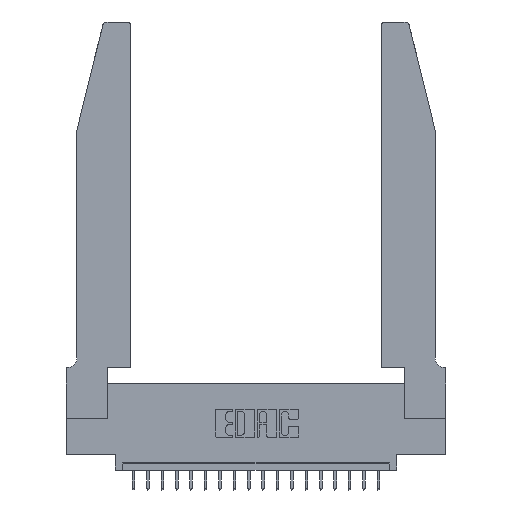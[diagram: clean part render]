
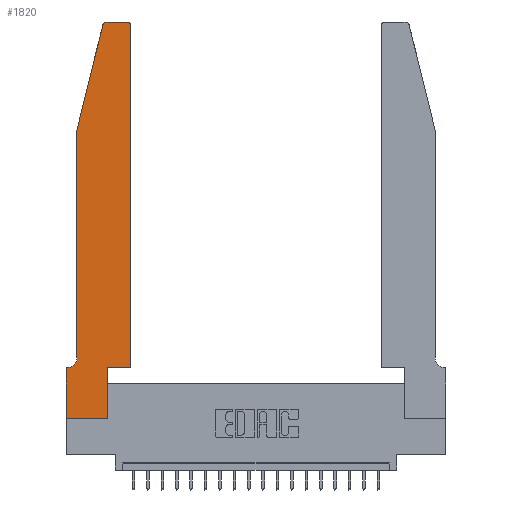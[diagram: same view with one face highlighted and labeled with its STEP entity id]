
A CAD part, top view. The second image highlights one B-rep face of the part: STEP entity #1820.
In plain terms, the highlighted planar face has unit normal (0, 0, 1).
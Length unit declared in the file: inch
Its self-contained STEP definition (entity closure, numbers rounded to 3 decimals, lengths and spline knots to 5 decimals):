
#83 = CARTESIAN_POINT ( 'NONE',  ( 0., 0., 0.37 ) ) ;
#143 = CARTESIAN_POINT ( 'NONE',  ( 0., 0.35, 0.37 ) ) ;
#421 = CARTESIAN_POINT ( 'NONE',  ( 0.0755, 0.42, 0.37 ) ) ;
#823 = CARTESIAN_POINT ( 'NONE',  ( 0.2605, 2.75, 0.37 ) ) ;
#1462 = VECTOR ( 'NONE', #4041, 39.37008 ) ;
#1718 = ORIENTED_EDGE ( 'NONE', *, *, #9220, .T. ) ;
#1743 = LINE ( 'NONE', #6698, #9475 ) ;
#1820 = ADVANCED_FACE ( 'NONE', ( #16213 ), #4867, .T. ) ;
#1913 = ORIENTED_EDGE ( 'NONE', *, *, #7084, .T. ) ;
#1983 = CARTESIAN_POINT ( 'NONE',  ( 0.2865, 0.35, 0.37 ) ) ;
#2235 = CARTESIAN_POINT ( 'NONE',  ( 0.284, 2.72, 0.37 ) ) ;
#2247 = VERTEX_POINT ( 'NONE', #15084 ) ;
#2311 = CARTESIAN_POINT ( 'NONE',  ( 0., 0., 0.37 ) ) ;
#2673 = AXIS2_PLACEMENT_3D ( 'NONE', #14909, #11725, #10182 ) ;
#2847 = CARTESIAN_POINT ( 'NONE',  ( 0.4505, 0.35, 0.37 ) ) ;
#3314 = ORIENTED_EDGE ( 'NONE', *, *, #6901, .T. ) ;
#3519 = VERTEX_POINT ( 'NONE', #1983 ) ;
#3571 = VECTOR ( 'NONE', #21142, 39.37008 ) ;
#3881 = CARTESIAN_POINT ( 'NONE',  ( 0.4505, 0.35, 0.37 ) ) ;
#4041 = DIRECTION ( 'NONE',  ( -1., 0., 0. ) ) ;
#4102 = CARTESIAN_POINT ( 'NONE',  ( 0.2865, 0., 0.37 ) ) ;
#4255 = CARTESIAN_POINT ( 'NONE',  ( 0.0055, 0.35, 0.37 ) ) ;
#4302 = LINE ( 'NONE', #5862, #3571 ) ;
#4397 = VERTEX_POINT ( 'NONE', #13463 ) ;
#4502 = CARTESIAN_POINT ( 'NONE',  ( 0.25487, 2.72718, 0.37 ) ) ;
#4761 = CARTESIAN_POINT ( 'NONE',  ( 0.0055, 0.42, 0.37 ) ) ;
#4792 = EDGE_CURVE ( 'NONE', #20558, #2247, #1743, .T. ) ;
#4867 = PLANE ( 'NONE',  #11579 ) ;
#5631 = VERTEX_POINT ( 'NONE', #143 ) ;
#5745 = LINE ( 'NONE', #7727, #11145 ) ;
#5862 = CARTESIAN_POINT ( 'NONE',  ( 0., 0., 0.37 ) ) ;
#5987 = DIRECTION ( 'NONE',  ( -1., 0., 0. ) ) ;
#6522 = VERTEX_POINT ( 'NONE', #421 ) ;
#6698 = CARTESIAN_POINT ( 'NONE',  ( 0.0755, 2., 0.37 ) ) ;
#6895 = EDGE_CURVE ( 'NONE', #7640, #20558, #8828, .T. ) ;
#6901 = EDGE_CURVE ( 'NONE', #14766, #4397, #20722, .T. ) ;
#7055 = ORIENTED_EDGE ( 'NONE', *, *, #10896, .T. ) ;
#7084 = EDGE_CURVE ( 'NONE', #19319, #17092, #4302, .T. ) ;
#7640 = VERTEX_POINT ( 'NONE', #21561 ) ;
#7681 = LINE ( 'NONE', #14392, #1462 ) ;
#7727 = CARTESIAN_POINT ( 'NONE',  ( 0.0755, 2., 0.37 ) ) ;
#7850 = DIRECTION ( 'NONE',  ( 0., 0., 1. ) ) ;
#7981 = ORIENTED_EDGE ( 'NONE', *, *, #12737, .T. ) ;
#8828 = CIRCLE ( 'NONE', #20438, 0.03 ) ;
#8900 = ORIENTED_EDGE ( 'NONE', *, *, #13479, .T. ) ;
#9220 = EDGE_CURVE ( 'NONE', #3519, #14766, #11209, .T. ) ;
#9347 = VECTOR ( 'NONE', #12766, 39.37008 ) ;
#9475 = VECTOR ( 'NONE', #16934, 39.37008 ) ;
#10182 = DIRECTION ( 'NONE',  ( 1., 0., 0. ) ) ;
#10896 = EDGE_CURVE ( 'NONE', #6522, #11415, #21543, .T. ) ;
#11086 = VECTOR ( 'NONE', #5987, 39.37008 ) ;
#11145 = VECTOR ( 'NONE', #14115, 39.37008 ) ;
#11209 = LINE ( 'NONE', #14274, #20149 ) ;
#11415 = VERTEX_POINT ( 'NONE', #4255 ) ;
#11483 = CARTESIAN_POINT ( 'NONE',  ( 0.2865, 0.35, 0.37 ) ) ;
#11579 = AXIS2_PLACEMENT_3D ( 'NONE', #16434, #7850, #11614 ) ;
#11614 = DIRECTION ( 'NONE',  ( 1., 0., 0. ) ) ;
#11725 = DIRECTION ( 'NONE',  ( 0., 0., 1. ) ) ;
#12327 = ORIENTED_EDGE ( 'NONE', *, *, #18652, .T. ) ;
#12737 = EDGE_CURVE ( 'NONE', #21011, #7640, #19208, .T. ) ;
#12766 = DIRECTION ( 'NONE',  ( 0., -1., 0. ) ) ;
#13421 = ORIENTED_EDGE ( 'NONE', *, *, #4792, .T. ) ;
#13431 = DIRECTION ( 'NONE',  ( 0., 1., 0. ) ) ;
#13463 = CARTESIAN_POINT ( 'NONE',  ( 0.4505, 2.72, 0.37 ) ) ;
#13479 = EDGE_CURVE ( 'NONE', #5631, #19319, #17497, .T. ) ;
#13539 = VECTOR ( 'NONE', #13431, 39.37008 ) ;
#13905 = DIRECTION ( 'NONE',  ( 1., 0., 0. ) ) ;
#13996 = EDGE_CURVE ( 'NONE', #4397, #21011, #16383, .T. ) ;
#14115 = DIRECTION ( 'NONE',  ( 0., -1., 0. ) ) ;
#14199 = EDGE_CURVE ( 'NONE', #2247, #6522, #5745, .T. ) ;
#14274 = CARTESIAN_POINT ( 'NONE',  ( 0.4505, 0.35, 0.37 ) ) ;
#14392 = CARTESIAN_POINT ( 'NONE',  ( 0.0755, 0.35, 0.37 ) ) ;
#14479 = DIRECTION ( 'NONE',  ( 1., 0., 0. ) ) ;
#14766 = VERTEX_POINT ( 'NONE', #2847 ) ;
#14909 = CARTESIAN_POINT ( 'NONE',  ( 0.4205, 2.72, 0.37 ) ) ;
#14918 = ORIENTED_EDGE ( 'NONE', *, *, #6895, .T. ) ;
#15040 = EDGE_CURVE ( 'NONE', #11415, #5631, #7681, .T. ) ;
#15084 = CARTESIAN_POINT ( 'NONE',  ( 0.0755, 2., 0.37 ) ) ;
#15106 = DIRECTION ( 'NONE',  ( -1., 0., 0. ) ) ;
#15506 = EDGE_LOOP ( 'NONE', ( #7981, #14918, #13421, #19414, #7055, #20627, #8900, #1913, #12327, #1718, #3314, #20055 ) ) ;
#16203 = VECTOR ( 'NONE', #20618, 39.37008 ) ;
#16213 = FACE_OUTER_BOUND ( 'NONE', #15506, .T. ) ;
#16383 = CIRCLE ( 'NONE', #2673, 0.03 ) ;
#16434 = CARTESIAN_POINT ( 'NONE',  ( 0., 0.35, 0.37 ) ) ;
#16934 = DIRECTION ( 'NONE',  ( -0.239, -0.971, 0. ) ) ;
#16995 = CARTESIAN_POINT ( 'NONE',  ( 0.4205, 2.75, 0.37 ) ) ;
#17092 = VERTEX_POINT ( 'NONE', #4102 ) ;
#17212 = DIRECTION ( 'NONE',  ( 0., 0., 1. ) ) ;
#17343 = AXIS2_PLACEMENT_3D ( 'NONE', #4761, #19722, #15106 ) ;
#17497 = LINE ( 'NONE', #2311, #9347 ) ;
#18652 = EDGE_CURVE ( 'NONE', #17092, #3519, #19376, .T. ) ;
#19208 = LINE ( 'NONE', #823, #11086 ) ;
#19319 = VERTEX_POINT ( 'NONE', #83 ) ;
#19376 = LINE ( 'NONE', #11483, #13539 ) ;
#19414 = ORIENTED_EDGE ( 'NONE', *, *, #14199, .T. ) ;
#19722 = DIRECTION ( 'NONE',  ( 0., 0., -1. ) ) ;
#20055 = ORIENTED_EDGE ( 'NONE', *, *, #13996, .T. ) ;
#20149 = VECTOR ( 'NONE', #14479, 39.37008 ) ;
#20438 = AXIS2_PLACEMENT_3D ( 'NONE', #2235, #17212, #13905 ) ;
#20558 = VERTEX_POINT ( 'NONE', #4502 ) ;
#20618 = DIRECTION ( 'NONE',  ( 0., 1., 0. ) ) ;
#20627 = ORIENTED_EDGE ( 'NONE', *, *, #15040, .T. ) ;
#20722 = LINE ( 'NONE', #3881, #16203 ) ;
#21011 = VERTEX_POINT ( 'NONE', #16995 ) ;
#21142 = DIRECTION ( 'NONE',  ( 1., 0., 0. ) ) ;
#21543 = CIRCLE ( 'NONE', #17343, 0.07 ) ;
#21561 = CARTESIAN_POINT ( 'NONE',  ( 0.284, 2.75, 0.37 ) ) ;
